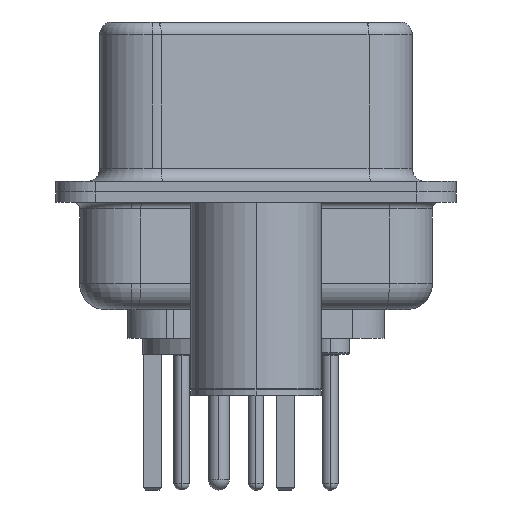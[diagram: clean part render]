
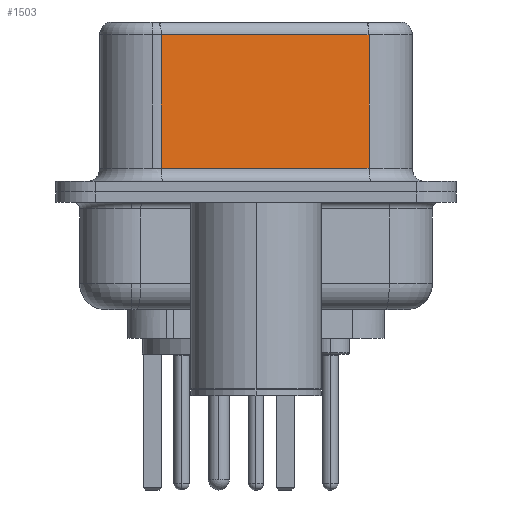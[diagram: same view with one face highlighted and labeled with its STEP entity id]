
A CAD part, left-side view. The second image highlights one B-rep face of the part: STEP entity #1503.
In plain terms, the highlighted planar face has unit normal (-0.985, -0.174, 0).
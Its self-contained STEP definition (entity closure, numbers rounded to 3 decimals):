
#423 = VERTEX_POINT ( 'NONE', #9581 ) ;
#914 = CARTESIAN_POINT ( 'NONE',  ( 3.73, 3.628, 6.52 ) ) ;
#1459 = EDGE_CURVE ( 'NONE', #16056, #17657, #6880, .T. ) ;
#1503 = ADVANCED_FACE ( 'NONE', ( #28302 ), #22700, .F. ) ;
#3135 = CARTESIAN_POINT ( 'NONE',  ( 5.132, -4.322, 6.02 ) ) ;
#5634 = CARTESIAN_POINT ( 'NONE',  ( 3.73, 3.628, 6.02 ) ) ;
#6880 = LINE ( 'NONE', #914, #16769 ) ;
#7846 = CARTESIAN_POINT ( 'NONE',  ( 5.132, -4.322, 6.52 ) ) ;
#8444 = ORIENTED_EDGE ( 'NONE', *, *, #13595, .F. ) ;
#9581 = CARTESIAN_POINT ( 'NONE',  ( 5.132, -4.322, 0.9 ) ) ;
#9751 = ORIENTED_EDGE ( 'NONE', *, *, #1459, .T. ) ;
#10021 = LINE ( 'NONE', #21505, #29001 ) ;
#11239 = EDGE_CURVE ( 'NONE', #14288, #16056, #10021, .T. ) ;
#12033 = CARTESIAN_POINT ( 'NONE',  ( 5.132, -4.322, 6.52 ) ) ;
#13595 = EDGE_CURVE ( 'NONE', #14288, #423, #28507, .T. ) ;
#14288 = VERTEX_POINT ( 'NONE', #3135 ) ;
#15585 = LINE ( 'NONE', #18372, #27126 ) ;
#16056 = VERTEX_POINT ( 'NONE', #5634 ) ;
#16769 = VECTOR ( 'NONE', #17936, 1000. ) ;
#16841 = AXIS2_PLACEMENT_3D ( 'NONE', #7846, #18631, #22739 ) ;
#17657 = VERTEX_POINT ( 'NONE', #24641 ) ;
#17704 = VECTOR ( 'NONE', #25744, 1000. ) ;
#17936 = DIRECTION ( 'NONE',  ( 0., 0., -1. ) ) ;
#18117 = ORIENTED_EDGE ( 'NONE', *, *, #11239, .T. ) ;
#18372 = CARTESIAN_POINT ( 'NONE',  ( 5.132, -4.322, 0.9 ) ) ;
#18631 = DIRECTION ( 'NONE',  ( 0.985, 0.174, 0. ) ) ;
#19081 = EDGE_LOOP ( 'NONE', ( #8444, #18117, #9751, #29476 ) ) ;
#19590 = EDGE_CURVE ( 'NONE', #17657, #423, #15585, .T. ) ;
#20754 = DIRECTION ( 'NONE',  ( 0.174, -0.985, 0. ) ) ;
#21505 = CARTESIAN_POINT ( 'NONE',  ( 5.132, -4.322, 6.02 ) ) ;
#22700 = PLANE ( 'NONE',  #16841 ) ;
#22739 = DIRECTION ( 'NONE',  ( -0.174, 0.985, 0. ) ) ;
#24641 = CARTESIAN_POINT ( 'NONE',  ( 3.73, 3.628, 0.9 ) ) ;
#25744 = DIRECTION ( 'NONE',  ( 0., 0., -1. ) ) ;
#25878 = DIRECTION ( 'NONE',  ( -0.174, 0.985, 0. ) ) ;
#27126 = VECTOR ( 'NONE', #20754, 1000. ) ;
#28302 = FACE_OUTER_BOUND ( 'NONE', #19081, .T. ) ;
#28507 = LINE ( 'NONE', #12033, #17704 ) ;
#29001 = VECTOR ( 'NONE', #25878, 1000. ) ;
#29476 = ORIENTED_EDGE ( 'NONE', *, *, #19590, .T. ) ;
